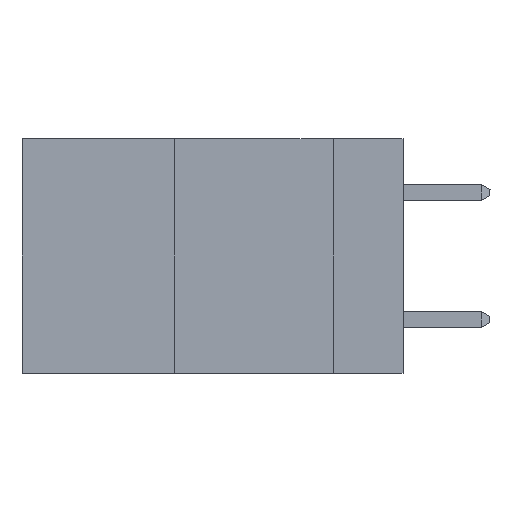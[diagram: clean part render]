
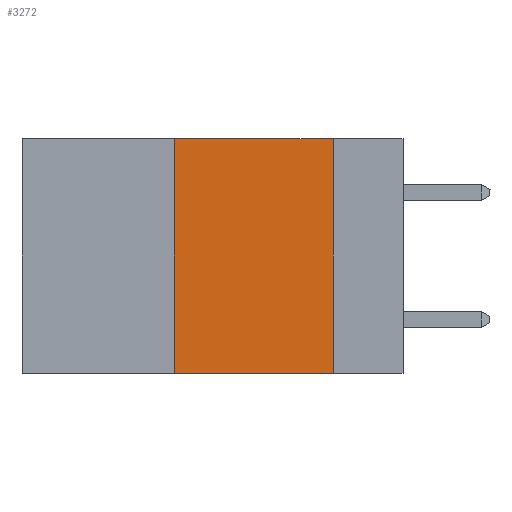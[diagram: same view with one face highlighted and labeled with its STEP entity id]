
A CAD part, left-side view. The second image highlights one B-rep face of the part: STEP entity #3272.
In plain terms, the highlighted planar face has unit normal (-1, 0, 0).
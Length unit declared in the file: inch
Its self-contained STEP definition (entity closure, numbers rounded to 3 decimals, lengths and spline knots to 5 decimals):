
#43 = CARTESIAN_POINT ( 'NONE',  ( 0., 0.6, -0.37 ) ) ;
#67 = VERTEX_POINT ( 'NONE', #13502 ) ;
#348 = LINE ( 'NONE', #43, #24699 ) ;
#1490 = CARTESIAN_POINT ( 'NONE',  ( 0., 0.11, 0. ) ) ;
#3272 = ADVANCED_FACE ( 'NONE', ( #18463 ), #27419, .F. ) ;
#3482 = DIRECTION ( 'NONE',  ( 0., 0., 1. ) ) ;
#4458 = DIRECTION ( 'NONE',  ( 0., 0., -1. ) ) ;
#4878 = VECTOR ( 'NONE', #14486, 39.37008 ) ;
#6202 = VERTEX_POINT ( 'NONE', #7388 ) ;
#6209 = ORIENTED_EDGE ( 'NONE', *, *, #11314, .F. ) ;
#7153 = CARTESIAN_POINT ( 'NONE',  ( 0., 0.36, 0. ) ) ;
#7318 = CARTESIAN_POINT ( 'NONE',  ( 0., 0.6, 0. ) ) ;
#7388 = CARTESIAN_POINT ( 'NONE',  ( 0., 0.36, 0. ) ) ;
#7456 = DIRECTION ( 'NONE',  ( 1., 0., 0. ) ) ;
#8121 = ORIENTED_EDGE ( 'NONE', *, *, #14606, .F. ) ;
#8578 = LINE ( 'NONE', #13259, #25444 ) ;
#9377 = CARTESIAN_POINT ( 'NONE',  ( 0., 0.6, 0. ) ) ;
#10199 = EDGE_CURVE ( 'NONE', #21993, #18379, #8578, .T. ) ;
#10569 = ORIENTED_EDGE ( 'NONE', *, *, #27121, .T. ) ;
#11314 = EDGE_CURVE ( 'NONE', #6202, #21993, #13774, .T. ) ;
#12825 = CARTESIAN_POINT ( 'NONE',  ( 0., 0.11, -0.37 ) ) ;
#13259 = CARTESIAN_POINT ( 'NONE',  ( 0., 0.11, 0. ) ) ;
#13502 = CARTESIAN_POINT ( 'NONE',  ( 0., 0.36, -0.37 ) ) ;
#13774 = LINE ( 'NONE', #9377, #4878 ) ;
#14486 = DIRECTION ( 'NONE',  ( 0., -1., 0. ) ) ;
#14606 = EDGE_CURVE ( 'NONE', #67, #6202, #27261, .T. ) ;
#17118 = AXIS2_PLACEMENT_3D ( 'NONE', #7318, #7456, #18312 ) ;
#18226 = DIRECTION ( 'NONE',  ( 0., -1., 0. ) ) ;
#18312 = DIRECTION ( 'NONE',  ( 0., 0., -1. ) ) ;
#18379 = VERTEX_POINT ( 'NONE', #12825 ) ;
#18463 = FACE_OUTER_BOUND ( 'NONE', #21331, .T. ) ;
#20397 = VECTOR ( 'NONE', #3482, 39.37008 ) ;
#21331 = EDGE_LOOP ( 'NONE', ( #28650, #6209, #8121, #10569 ) ) ;
#21993 = VERTEX_POINT ( 'NONE', #1490 ) ;
#24699 = VECTOR ( 'NONE', #18226, 39.37008 ) ;
#25444 = VECTOR ( 'NONE', #4458, 39.37008 ) ;
#27121 = EDGE_CURVE ( 'NONE', #67, #18379, #348, .T. ) ;
#27261 = LINE ( 'NONE', #7153, #20397 ) ;
#27419 = PLANE ( 'NONE',  #17118 ) ;
#28650 = ORIENTED_EDGE ( 'NONE', *, *, #10199, .F. ) ;
